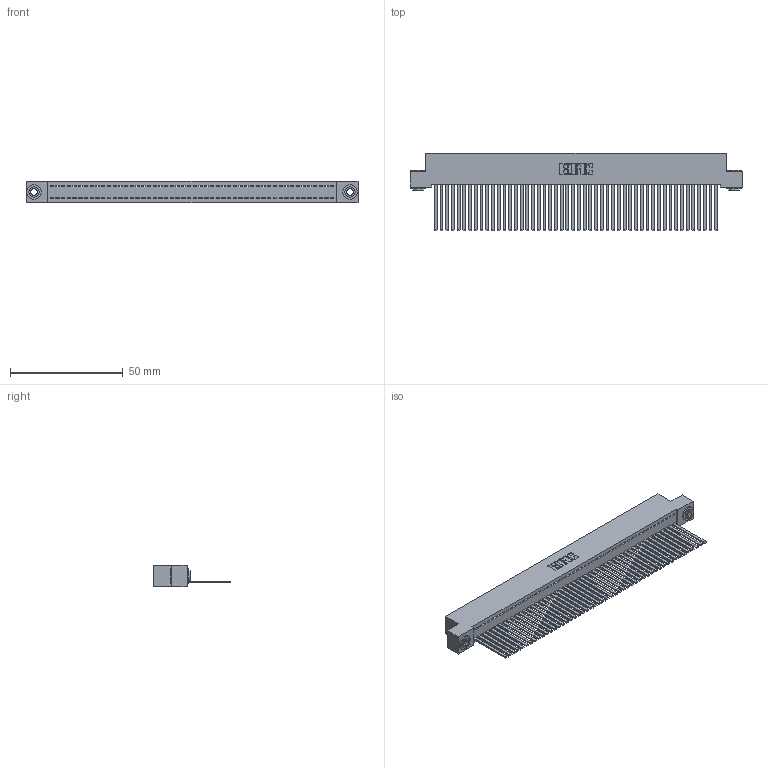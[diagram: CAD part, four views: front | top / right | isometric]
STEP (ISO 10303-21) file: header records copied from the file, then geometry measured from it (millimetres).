
FILE_DESCRIPTION (( 'STEP AP203' ), '1' );
FILE_NAME ('342-050-544-103.STEP', '2019-10-02T23:51:09', ( '' ), ( '' ), 'SwSTEP 2.0', 'SolidWorks 2016', '' );
FILE_SCHEMA (( 'CONFIG_CONTROL_DESIGN' ));
Length unit declared in the file: inch
Products named in the file (4): 342 Part_.156 TH; 345-292-001_345-293-144; 342-250-002_345-250-002-102; 342-050-544-103
Assembly tree (53 placements, depth 2):
  342-050-544-103
    342 Part_.156 TH
    345-292-001_345-293-144  x50
    342-250-002_345-250-002-102  x2
Bounding box: 147.32 x 34.3 x 9.4 mm (x, y, z)
Volume: 13548.4 mm3; surface area: 21918.8 mm2
Topology: 53 solids, 53 shells, 2748 faces, 8275 edges, 5446 vertices
Faces by surface type: plane 1976, cylinder 764, cone 8
Entity records: 29866 total; most frequent: CARTESIAN_POINT 5127, ORIENTED_EDGE 5106, DIRECTION 4339, EDGE_CURVE 2553, VECTOR 2405, LINE 2405, VERTEX_POINT 1698, AXIS2_PLACEMENT_3D 967
